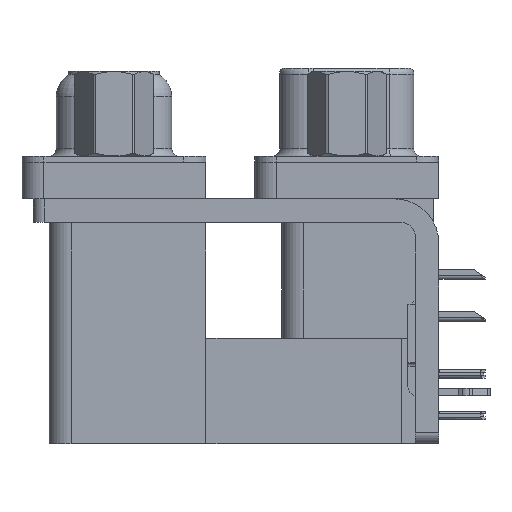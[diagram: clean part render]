
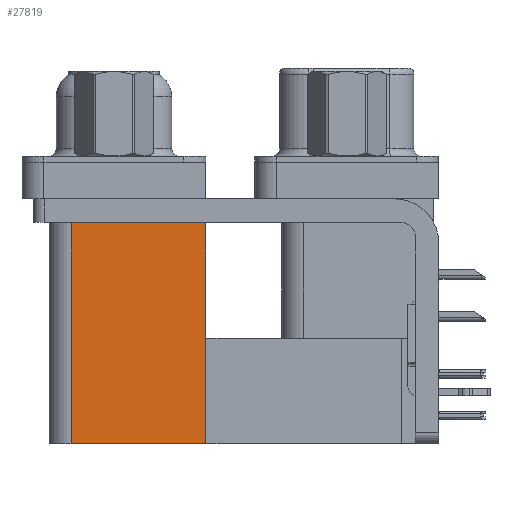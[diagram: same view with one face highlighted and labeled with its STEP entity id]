
A CAD part, left-side view. The second image highlights one B-rep face of the part: STEP entity #27819.
In plain terms, the highlighted planar face has unit normal (-1, 0, 0).
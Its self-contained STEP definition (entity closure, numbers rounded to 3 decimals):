
#215 = AXIS2_PLACEMENT_3D ( 'NONE', #41794, #49249, #3021 ) ;
#3021 = DIRECTION ( 'NONE',  ( 0., 0., -1. ) ) ;
#4483 = DIRECTION ( 'NONE',  ( 0., 0., 1. ) ) ;
#7204 = CARTESIAN_POINT ( 'NONE',  ( 3.765, 9.6, -2.5 ) ) ;
#7541 = LINE ( 'NONE', #42959, #34089 ) ;
#11507 = VERTEX_POINT ( 'NONE', #38240 ) ;
#11747 = VECTOR ( 'NONE', #4483, 1000. ) ;
#15285 = LINE ( 'NONE', #35027, #11747 ) ;
#18330 = LINE ( 'NONE', #25033, #28591 ) ;
#18470 = VECTOR ( 'NONE', #45210, 1000. ) ;
#18915 = EDGE_CURVE ( 'NONE', #36157, #34214, #18330, .T. ) ;
#20180 = ORIENTED_EDGE ( 'NONE', *, *, #18915, .F. ) ;
#20471 = VERTEX_POINT ( 'NONE', #34746 ) ;
#23031 = PLANE ( 'NONE',  #215 ) ;
#25033 = CARTESIAN_POINT ( 'NONE',  ( 3.765, 9.6, -19.2 ) ) ;
#26378 = FACE_OUTER_BOUND ( 'NONE', #43388, .T. ) ;
#27016 = ORIENTED_EDGE ( 'NONE', *, *, #28350, .F. ) ;
#27662 = ORIENTED_EDGE ( 'NONE', *, *, #42461, .T. ) ;
#27819 = ADVANCED_FACE ( 'NONE', ( #26378 ), #23031, .F. ) ;
#28026 = DIRECTION ( 'NONE',  ( 0., 0., 1. ) ) ;
#28350 = EDGE_CURVE ( 'NONE', #34214, #11507, #15285, .T. ) ;
#28591 = VECTOR ( 'NONE', #29861, 1000. ) ;
#29861 = DIRECTION ( 'NONE',  ( 0., 1., 0. ) ) ;
#34089 = VECTOR ( 'NONE', #28026, 1000. ) ;
#34214 = VERTEX_POINT ( 'NONE', #39343 ) ;
#34285 = EDGE_CURVE ( 'NONE', #36157, #20471, #7541, .T. ) ;
#34746 = CARTESIAN_POINT ( 'NONE',  ( 3.765, 9.6, -2.5 ) ) ;
#35027 = CARTESIAN_POINT ( 'NONE',  ( 3.765, 18.8, -19.2 ) ) ;
#36157 = VERTEX_POINT ( 'NONE', #37220 ) ;
#37220 = CARTESIAN_POINT ( 'NONE',  ( 3.765, 9.6, -19.2 ) ) ;
#38240 = CARTESIAN_POINT ( 'NONE',  ( 3.765, 18.8, -2.5 ) ) ;
#39343 = CARTESIAN_POINT ( 'NONE',  ( 3.765, 18.8, -19.2 ) ) ;
#41794 = CARTESIAN_POINT ( 'NONE',  ( 3.765, 9.6, -19.2 ) ) ;
#42165 = ORIENTED_EDGE ( 'NONE', *, *, #34285, .T. ) ;
#42461 = EDGE_CURVE ( 'NONE', #20471, #11507, #46208, .T. ) ;
#42959 = CARTESIAN_POINT ( 'NONE',  ( 3.765, 9.6, -19.2 ) ) ;
#43388 = EDGE_LOOP ( 'NONE', ( #27662, #27016, #20180, #42165 ) ) ;
#45210 = DIRECTION ( 'NONE',  ( 0., 1., 0. ) ) ;
#46208 = LINE ( 'NONE', #7204, #18470 ) ;
#49249 = DIRECTION ( 'NONE',  ( 1., 0., 0. ) ) ;
